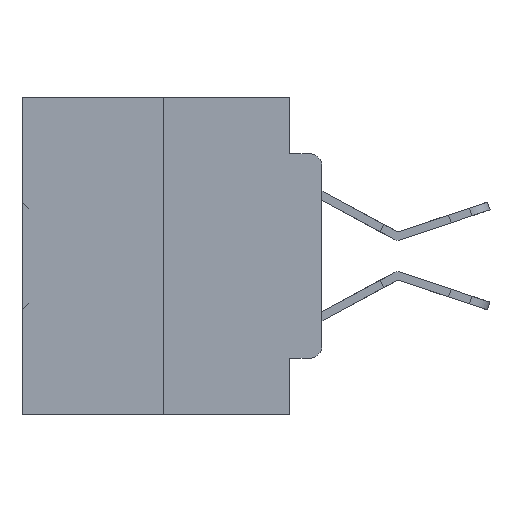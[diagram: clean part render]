
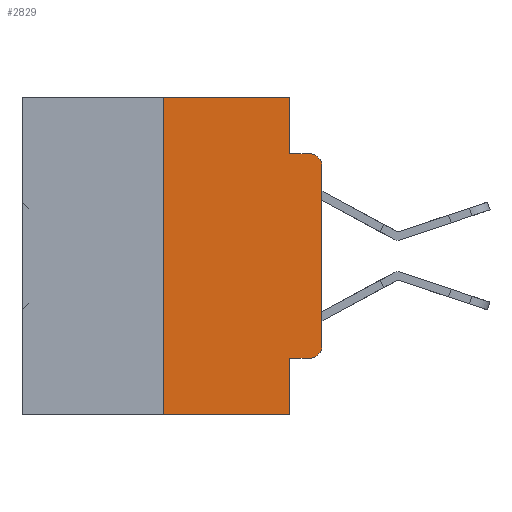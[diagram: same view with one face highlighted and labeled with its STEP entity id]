
A CAD part, left-side view. The second image highlights one B-rep face of the part: STEP entity #2829.
In plain terms, the highlighted planar face has unit normal (-1, 0, 0).
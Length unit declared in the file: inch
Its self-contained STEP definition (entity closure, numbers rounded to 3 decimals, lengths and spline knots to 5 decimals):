
#934 = EDGE_CURVE ( 'NONE', #22553, #19976, #25992, .T. ) ;
#956 = DIRECTION ( 'NONE',  ( 0., -1., 0. ) ) ;
#2388 = EDGE_CURVE ( 'NONE', #30809, #22553, #27777, .T. ) ;
#2702 = LINE ( 'NONE', #6022, #39053 ) ;
#2829 = ADVANCED_FACE ( 'NONE', ( #4593 ), #28475, .F. ) ;
#2843 = ORIENTED_EDGE ( 'NONE', *, *, #13634, .F. ) ;
#3933 = DIRECTION ( 'NONE',  ( 0., 0., -1. ) ) ;
#4132 = VERTEX_POINT ( 'NONE', #5183 ) ;
#4593 = FACE_OUTER_BOUND ( 'NONE', #31008, .T. ) ;
#5183 = CARTESIAN_POINT ( 'NONE',  ( 0., 0., -0.1085 ) ) ;
#5220 = CARTESIAN_POINT ( 'NONE',  ( 0., 0., 0. ) ) ;
#5277 = CIRCLE ( 'NONE', #11058, 0.02 ) ;
#6022 = CARTESIAN_POINT ( 'NONE',  ( 0., 0.051, 0. ) ) ;
#6820 = CIRCLE ( 'NONE', #22570, 0.02 ) ;
#6903 = DIRECTION ( 'NONE',  ( 0., 0., 1. ) ) ;
#8419 = DIRECTION ( 'NONE',  ( 0., -1., 0. ) ) ;
#8592 = VERTEX_POINT ( 'NONE', #27600 ) ;
#8630 = CARTESIAN_POINT ( 'NONE',  ( 0., 0.051, 0. ) ) ;
#9401 = VECTOR ( 'NONE', #6903, 39.37008 ) ;
#9547 = EDGE_CURVE ( 'NONE', #8592, #4132, #21462, .T. ) ;
#9558 = CARTESIAN_POINT ( 'NONE',  ( 0., 0.051, 0. ) ) ;
#9687 = VERTEX_POINT ( 'NONE', #33007 ) ;
#9938 = EDGE_CURVE ( 'NONE', #4132, #27552, #5277, .T. ) ;
#10430 = ORIENTED_EDGE ( 'NONE', *, *, #934, .F. ) ;
#11058 = AXIS2_PLACEMENT_3D ( 'NONE', #19419, #34281, #3933 ) ;
#11724 = CARTESIAN_POINT ( 'NONE',  ( 0., 0.051, -0.0885 ) ) ;
#11779 = VECTOR ( 'NONE', #15627, 39.37008 ) ;
#12096 = CARTESIAN_POINT ( 'NONE',  ( 0., 0.051, -0.0885 ) ) ;
#12421 = VECTOR ( 'NONE', #29424, 39.37008 ) ;
#12441 = ORIENTED_EDGE ( 'NONE', *, *, #33648, .F. ) ;
#12628 = VECTOR ( 'NONE', #8419, 39.37008 ) ;
#13396 = CARTESIAN_POINT ( 'NONE',  ( 0., 0.473, 0. ) ) ;
#13634 = EDGE_CURVE ( 'NONE', #21458, #31307, #2702, .T. ) ;
#14222 = AXIS2_PLACEMENT_3D ( 'NONE', #13396, #16688, #22586 ) ;
#14933 = DIRECTION ( 'NONE',  ( 0., 0., -1. ) ) ;
#15627 = DIRECTION ( 'NONE',  ( 0., 0., -1. ) ) ;
#16688 = DIRECTION ( 'NONE',  ( 1., 0., 0. ) ) ;
#17268 = ORIENTED_EDGE ( 'NONE', *, *, #17827, .T. ) ;
#17789 = CARTESIAN_POINT ( 'NONE',  ( 0., 0.051, -0.4115 ) ) ;
#17827 = EDGE_CURVE ( 'NONE', #21458, #9687, #38000, .T. ) ;
#18192 = CARTESIAN_POINT ( 'NONE',  ( 0., 0.02, -0.0885 ) ) ;
#19038 = CARTESIAN_POINT ( 'NONE',  ( 0., 0.25, 0. ) ) ;
#19039 = CARTESIAN_POINT ( 'NONE',  ( 0., 0.473, -0.5 ) ) ;
#19419 = CARTESIAN_POINT ( 'NONE',  ( 0., 0.02, -0.1085 ) ) ;
#19488 = EDGE_CURVE ( 'NONE', #34043, #31307, #33126, .T. ) ;
#19976 = VERTEX_POINT ( 'NONE', #12096 ) ;
#20876 = DIRECTION ( 'NONE',  ( 0., 0., -1. ) ) ;
#21458 = VERTEX_POINT ( 'NONE', #38003 ) ;
#21462 = LINE ( 'NONE', #5220, #28014 ) ;
#22553 = VERTEX_POINT ( 'NONE', #8630 ) ;
#22570 = AXIS2_PLACEMENT_3D ( 'NONE', #36840, #23843, #14933 ) ;
#22586 = DIRECTION ( 'NONE',  ( 0., 0., -1. ) ) ;
#22874 = VECTOR ( 'NONE', #956, 39.37008 ) ;
#22940 = CARTESIAN_POINT ( 'NONE',  ( 0., 0.25, -0.5 ) ) ;
#23843 = DIRECTION ( 'NONE',  ( -1., 0., 0. ) ) ;
#25269 = VECTOR ( 'NONE', #27034, 39.37008 ) ;
#25992 = LINE ( 'NONE', #9558, #11779 ) ;
#26664 = ORIENTED_EDGE ( 'NONE', *, *, #30092, .F. ) ;
#26977 = CARTESIAN_POINT ( 'NONE',  ( 0., 0.051, -0.5 ) ) ;
#27034 = DIRECTION ( 'NONE',  ( 0., -1., 0. ) ) ;
#27552 = VERTEX_POINT ( 'NONE', #18192 ) ;
#27600 = CARTESIAN_POINT ( 'NONE',  ( 0., 0., -0.3915 ) ) ;
#27667 = CARTESIAN_POINT ( 'NONE',  ( 0., 0.25, 0. ) ) ;
#27777 = LINE ( 'NONE', #38782, #12628 ) ;
#28014 = VECTOR ( 'NONE', #32437, 39.37008 ) ;
#28286 = ORIENTED_EDGE ( 'NONE', *, *, #19488, .T. ) ;
#28475 = PLANE ( 'NONE',  #14222 ) ;
#29424 = DIRECTION ( 'NONE',  ( 0., -1., 0. ) ) ;
#29471 = ORIENTED_EDGE ( 'NONE', *, *, #9938, .T. ) ;
#30092 = EDGE_CURVE ( 'NONE', #34043, #30809, #30653, .T. ) ;
#30653 = LINE ( 'NONE', #27667, #9401 ) ;
#30809 = VERTEX_POINT ( 'NONE', #19038 ) ;
#31008 = EDGE_LOOP ( 'NONE', ( #32433, #29471, #12441, #10430, #35939, #26664, #28286, #2843, #17268, #36473 ) ) ;
#31307 = VERTEX_POINT ( 'NONE', #26977 ) ;
#32268 = LINE ( 'NONE', #11724, #12421 ) ;
#32433 = ORIENTED_EDGE ( 'NONE', *, *, #9547, .T. ) ;
#32437 = DIRECTION ( 'NONE',  ( 0., 0., 1. ) ) ;
#33007 = CARTESIAN_POINT ( 'NONE',  ( 0., 0.02, -0.4115 ) ) ;
#33126 = LINE ( 'NONE', #19039, #22874 ) ;
#33648 = EDGE_CURVE ( 'NONE', #19976, #27552, #32268, .T. ) ;
#34043 = VERTEX_POINT ( 'NONE', #22940 ) ;
#34281 = DIRECTION ( 'NONE',  ( -1., 0., 0. ) ) ;
#35939 = ORIENTED_EDGE ( 'NONE', *, *, #2388, .F. ) ;
#36473 = ORIENTED_EDGE ( 'NONE', *, *, #36979, .T. ) ;
#36840 = CARTESIAN_POINT ( 'NONE',  ( 0., 0.02, -0.3915 ) ) ;
#36979 = EDGE_CURVE ( 'NONE', #9687, #8592, #6820, .T. ) ;
#38000 = LINE ( 'NONE', #17789, #25269 ) ;
#38003 = CARTESIAN_POINT ( 'NONE',  ( 0., 0.051, -0.4115 ) ) ;
#38782 = CARTESIAN_POINT ( 'NONE',  ( 0., 0.473, 0. ) ) ;
#39053 = VECTOR ( 'NONE', #20876, 39.37008 ) ;
